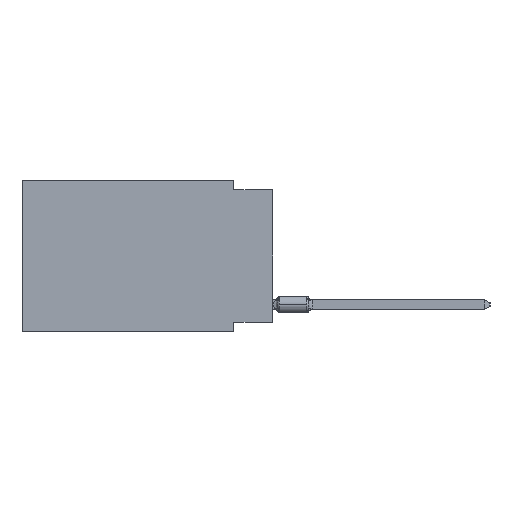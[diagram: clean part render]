
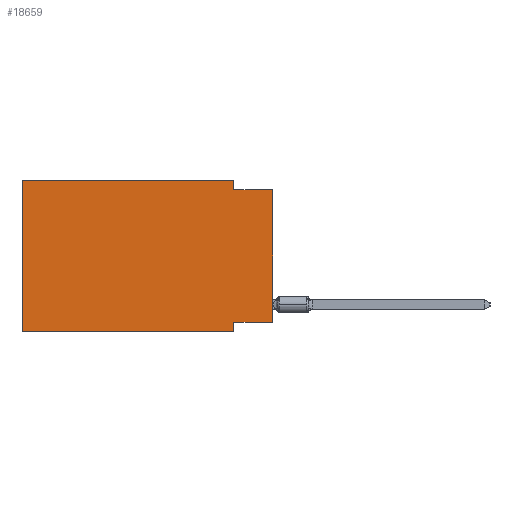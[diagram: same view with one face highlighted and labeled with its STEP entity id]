
A CAD part, left-side view. The second image highlights one B-rep face of the part: STEP entity #18659.
In plain terms, the highlighted planar face has unit normal (-1, 0, 0).
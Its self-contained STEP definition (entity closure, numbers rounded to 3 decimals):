
#56 = VERTEX_POINT ( 'NONE', #20056 ) ;
#110 = VECTOR ( 'NONE', #23776, 1000. ) ;
#610 = VECTOR ( 'NONE', #28910, 1000. ) ;
#1249 = FACE_OUTER_BOUND ( 'NONE', #24204, .T. ) ;
#1282 = CARTESIAN_POINT ( 'NONE',  ( 0., 0., 0. ) ) ;
#1374 = LINE ( 'NONE', #5380, #22807 ) ;
#1932 = LINE ( 'NONE', #8744, #18191 ) ;
#2483 = ORIENTED_EDGE ( 'NONE', *, *, #8336, .F. ) ;
#2530 = ORIENTED_EDGE ( 'NONE', *, *, #24776, .F. ) ;
#3219 = DIRECTION ( 'NONE',  ( 0., 0., 1. ) ) ;
#3327 = PLANE ( 'NONE',  #14752 ) ;
#4001 = VERTEX_POINT ( 'NONE', #22437 ) ;
#4808 = EDGE_CURVE ( 'NONE', #23619, #23812, #1932, .T. ) ;
#4925 = VERTEX_POINT ( 'NONE', #10657 ) ;
#5380 = CARTESIAN_POINT ( 'NONE',  ( 0., 16.383, 0. ) ) ;
#5540 = DIRECTION ( 'NONE',  ( 1., 0., 0. ) ) ;
#6319 = VERTEX_POINT ( 'NONE', #27533 ) ;
#6437 = VECTOR ( 'NONE', #3219, 1000. ) ;
#7017 = DIRECTION ( 'NONE',  ( 0., 0., -1. ) ) ;
#8336 = EDGE_CURVE ( 'NONE', #11080, #6319, #28551, .T. ) ;
#8452 = CARTESIAN_POINT ( 'NONE',  ( 0., 0., -0.635 ) ) ;
#8744 = CARTESIAN_POINT ( 'NONE',  ( 0., 0., -9.271 ) ) ;
#9027 = DIRECTION ( 'NONE',  ( 0., 1., 0. ) ) ;
#9051 = ORIENTED_EDGE ( 'NONE', *, *, #13666, .F. ) ;
#9238 = LINE ( 'NONE', #27260, #9761 ) ;
#9761 = VECTOR ( 'NONE', #7017, 1000. ) ;
#10657 = CARTESIAN_POINT ( 'NONE',  ( 0., 2.54, 0. ) ) ;
#11080 = VERTEX_POINT ( 'NONE', #23682 ) ;
#11365 = ORIENTED_EDGE ( 'NONE', *, *, #15358, .F. ) ;
#12202 = CARTESIAN_POINT ( 'NONE',  ( 0., 2.54, -9.271 ) ) ;
#12687 = CARTESIAN_POINT ( 'NONE',  ( 0., 16.383, -9.906 ) ) ;
#13666 = EDGE_CURVE ( 'NONE', #23812, #4001, #17530, .T. ) ;
#14398 = DIRECTION ( 'NONE',  ( 0., -1., 0. ) ) ;
#14752 = AXIS2_PLACEMENT_3D ( 'NONE', #19407, #5540, #28284 ) ;
#14783 = ORIENTED_EDGE ( 'NONE', *, *, #4808, .F. ) ;
#15169 = CARTESIAN_POINT ( 'NONE',  ( 0., 2.54, -9.906 ) ) ;
#15358 = EDGE_CURVE ( 'NONE', #4925, #11080, #9238, .T. ) ;
#16424 = VECTOR ( 'NONE', #26181, 1000. ) ;
#16520 = ORIENTED_EDGE ( 'NONE', *, *, #24328, .F. ) ;
#17300 = CARTESIAN_POINT ( 'NONE',  ( 0., 16.383, 0. ) ) ;
#17307 = ORIENTED_EDGE ( 'NONE', *, *, #18254, .T. ) ;
#17530 = LINE ( 'NONE', #15169, #610 ) ;
#17762 = ORIENTED_EDGE ( 'NONE', *, *, #23311, .T. ) ;
#18191 = VECTOR ( 'NONE', #9027, 1000. ) ;
#18254 = EDGE_CURVE ( 'NONE', #23619, #6319, #23744, .T. ) ;
#18659 = ADVANCED_FACE ( 'NONE', ( #1249 ), #3327, .F. ) ;
#19407 = CARTESIAN_POINT ( 'NONE',  ( 0., 16.383, 0. ) ) ;
#19501 = VECTOR ( 'NONE', #20355, 1000. ) ;
#20056 = CARTESIAN_POINT ( 'NONE',  ( 0., 16.383, 0. ) ) ;
#20355 = DIRECTION ( 'NONE',  ( 0., 0., 1. ) ) ;
#21864 = LINE ( 'NONE', #17300, #19501 ) ;
#22437 = CARTESIAN_POINT ( 'NONE',  ( 0., 2.54, -9.906 ) ) ;
#22807 = VECTOR ( 'NONE', #14398, 1000. ) ;
#23311 = EDGE_CURVE ( 'NONE', #27489, #4001, #23924, .T. ) ;
#23619 = VERTEX_POINT ( 'NONE', #29077 ) ;
#23682 = CARTESIAN_POINT ( 'NONE',  ( 0., 2.54, -0.635 ) ) ;
#23744 = LINE ( 'NONE', #1282, #6437 ) ;
#23776 = DIRECTION ( 'NONE',  ( 0., -1., 0. ) ) ;
#23812 = VERTEX_POINT ( 'NONE', #12202 ) ;
#23924 = LINE ( 'NONE', #12687, #110 ) ;
#24204 = EDGE_LOOP ( 'NONE', ( #17307, #2483, #11365, #16520, #2530, #17762, #9051, #14783 ) ) ;
#24328 = EDGE_CURVE ( 'NONE', #56, #4925, #1374, .T. ) ;
#24776 = EDGE_CURVE ( 'NONE', #27489, #56, #21864, .T. ) ;
#26181 = DIRECTION ( 'NONE',  ( 0., -1., 0. ) ) ;
#26888 = CARTESIAN_POINT ( 'NONE',  ( 0., 16.383, -9.906 ) ) ;
#27260 = CARTESIAN_POINT ( 'NONE',  ( 0., 2.54, 0. ) ) ;
#27489 = VERTEX_POINT ( 'NONE', #26888 ) ;
#27533 = CARTESIAN_POINT ( 'NONE',  ( 0., 0., -0.635 ) ) ;
#28284 = DIRECTION ( 'NONE',  ( 0., 0., -1. ) ) ;
#28551 = LINE ( 'NONE', #8452, #16424 ) ;
#28910 = DIRECTION ( 'NONE',  ( 0., 0., -1. ) ) ;
#29077 = CARTESIAN_POINT ( 'NONE',  ( 0., 0., -9.271 ) ) ;
